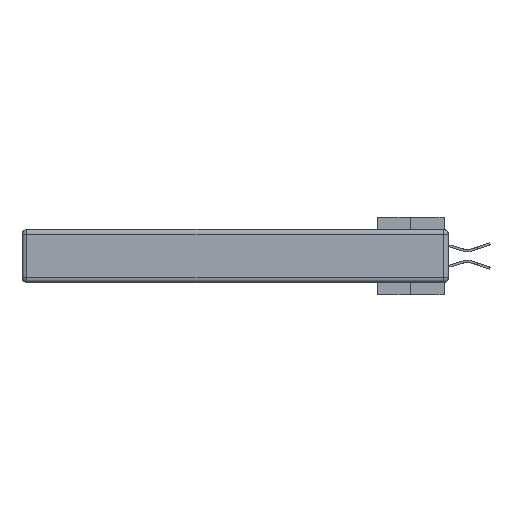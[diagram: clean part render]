
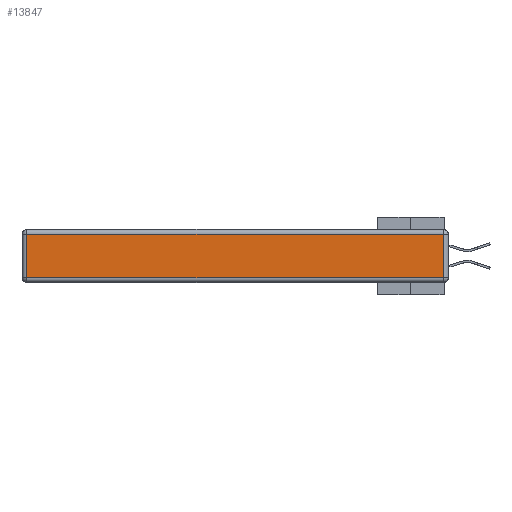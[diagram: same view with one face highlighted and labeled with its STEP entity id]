
A CAD part, left-side view. The second image highlights one B-rep face of the part: STEP entity #13847.
In plain terms, the highlighted planar face has unit normal (-1, 0, 0).
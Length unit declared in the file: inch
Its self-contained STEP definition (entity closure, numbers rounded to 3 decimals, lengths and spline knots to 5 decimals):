
#341 = VERTEX_POINT ( 'NONE', #11602 ) ;
#782 = ORIENTED_EDGE ( 'NONE', *, *, #20979, .T. ) ;
#1003 = EDGE_CURVE ( 'NONE', #31126, #28298, #9323, .T. ) ;
#2315 = DIRECTION ( 'NONE',  ( -1., 0., 0. ) ) ;
#4524 = CARTESIAN_POINT ( 'NONE',  ( 0., 0.03, -0.03 ) ) ;
#4709 = AXIS2_PLACEMENT_3D ( 'NONE', #20935, #2315, #21065 ) ;
#6117 = VERTEX_POINT ( 'NONE', #23674 ) ;
#7463 = DIRECTION ( 'NONE',  ( 0., 0., 1. ) ) ;
#9282 = DIRECTION ( 'NONE',  ( 0., 1., 0. ) ) ;
#9323 = LINE ( 'NONE', #27810, #28702 ) ;
#10495 = LINE ( 'NONE', #34099, #14378 ) ;
#11602 = CARTESIAN_POINT ( 'NONE',  ( 0., 0.03, -0.313 ) ) ;
#13847 = ADVANCED_FACE ( 'NONE', ( #38660 ), #15118, .T. ) ;
#14378 = VECTOR ( 'NONE', #26371, 39.37008 ) ;
#15118 = PLANE ( 'NONE',  #4709 ) ;
#16281 = CARTESIAN_POINT ( 'NONE',  ( 0., 0., -0.313 ) ) ;
#16313 = EDGE_LOOP ( 'NONE', ( #20897, #38056, #32965, #782 ) ) ;
#16629 = EDGE_CURVE ( 'NONE', #341, #31126, #24876, .T. ) ;
#16657 = CARTESIAN_POINT ( 'NONE',  ( 0., 0.03, -0.343 ) ) ;
#20897 = ORIENTED_EDGE ( 'NONE', *, *, #30377, .T. ) ;
#20935 = CARTESIAN_POINT ( 'NONE',  ( 0., 0., -0.343 ) ) ;
#20979 = EDGE_CURVE ( 'NONE', #28298, #6117, #10495, .T. ) ;
#21065 = DIRECTION ( 'NONE',  ( 0., 0., 1. ) ) ;
#21746 = VECTOR ( 'NONE', #31455, 39.37008 ) ;
#21955 = VECTOR ( 'NONE', #7463, 39.37008 ) ;
#23674 = CARTESIAN_POINT ( 'NONE',  ( 0., 2.72, -0.313 ) ) ;
#24876 = LINE ( 'NONE', #16657, #21955 ) ;
#26371 = DIRECTION ( 'NONE',  ( 0., 0., -1. ) ) ;
#27810 = CARTESIAN_POINT ( 'NONE',  ( 0., 2.75, -0.03 ) ) ;
#28298 = VERTEX_POINT ( 'NONE', #30329 ) ;
#28702 = VECTOR ( 'NONE', #9282, 39.37008 ) ;
#29974 = LINE ( 'NONE', #16281, #21746 ) ;
#30329 = CARTESIAN_POINT ( 'NONE',  ( 0., 2.72, -0.03 ) ) ;
#30377 = EDGE_CURVE ( 'NONE', #6117, #341, #29974, .T. ) ;
#31126 = VERTEX_POINT ( 'NONE', #4524 ) ;
#31455 = DIRECTION ( 'NONE',  ( 0., -1., 0. ) ) ;
#32965 = ORIENTED_EDGE ( 'NONE', *, *, #1003, .T. ) ;
#34099 = CARTESIAN_POINT ( 'NONE',  ( 0., 2.72, -0.343 ) ) ;
#38056 = ORIENTED_EDGE ( 'NONE', *, *, #16629, .T. ) ;
#38660 = FACE_OUTER_BOUND ( 'NONE', #16313, .T. ) ;
